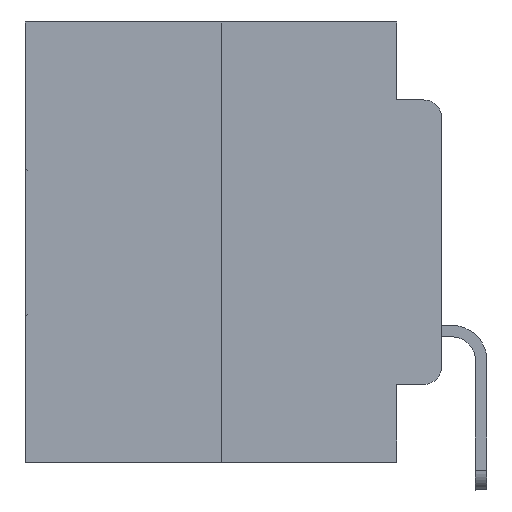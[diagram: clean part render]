
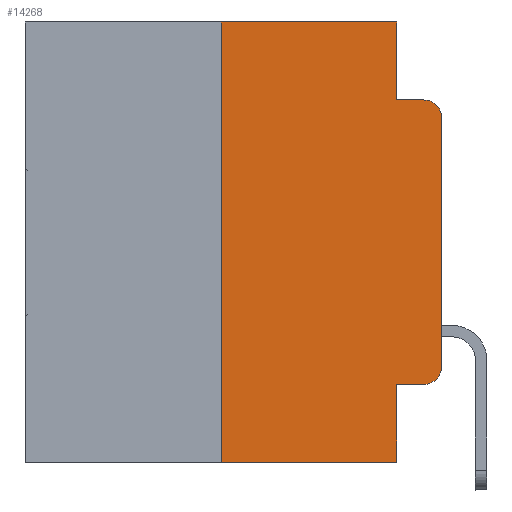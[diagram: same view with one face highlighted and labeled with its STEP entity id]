
A CAD part, left-side view. The second image highlights one B-rep face of the part: STEP entity #14268.
In plain terms, the highlighted planar face has unit normal (-1, 0, 0).
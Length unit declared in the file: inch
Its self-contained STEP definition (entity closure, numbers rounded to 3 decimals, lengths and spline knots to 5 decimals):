
#371 = LINE ( 'NONE', #25552, #9766 ) ;
#422 = CIRCLE ( 'NONE', #6718, 0.02 ) ;
#519 = EDGE_CURVE ( 'NONE', #29199, #28225, #18286, .T. ) ;
#1461 = EDGE_CURVE ( 'NONE', #24950, #4144, #371, .T. ) ;
#1488 = ORIENTED_EDGE ( 'NONE', *, *, #13376, .F. ) ;
#2342 = VECTOR ( 'NONE', #18894, 39.37008 ) ;
#2504 = DIRECTION ( 'NONE',  ( 0., -1., 0. ) ) ;
#2719 = CARTESIAN_POINT ( 'NONE',  ( 0., 0.051, 0. ) ) ;
#3191 = EDGE_CURVE ( 'NONE', #14461, #8366, #22677, .T. ) ;
#3916 = AXIS2_PLACEMENT_3D ( 'NONE', #18688, #4419, #9280 ) ;
#3962 = LINE ( 'NONE', #22178, #16787 ) ;
#4144 = VERTEX_POINT ( 'NONE', #12081 ) ;
#4322 = ORIENTED_EDGE ( 'NONE', *, *, #3191, .F. ) ;
#4419 = DIRECTION ( 'NONE',  ( 1., 0., 0. ) ) ;
#4584 = LINE ( 'NONE', #27183, #28174 ) ;
#5077 = LINE ( 'NONE', #18300, #29204 ) ;
#6096 = DIRECTION ( 'NONE',  ( 0., -1., 0. ) ) ;
#6636 = DIRECTION ( 'NONE',  ( 0., 0., 1. ) ) ;
#6718 = AXIS2_PLACEMENT_3D ( 'NONE', #18452, #28140, #27697 ) ;
#7083 = CARTESIAN_POINT ( 'NONE',  ( 0., 0.051, 0. ) ) ;
#7108 = VERTEX_POINT ( 'NONE', #17450 ) ;
#7921 = ORIENTED_EDGE ( 'NONE', *, *, #13433, .T. ) ;
#8366 = VERTEX_POINT ( 'NONE', #10190 ) ;
#8393 = CARTESIAN_POINT ( 'NONE',  ( 0., 0.02, -0.3915 ) ) ;
#8865 = VECTOR ( 'NONE', #11462, 39.37008 ) ;
#9280 = DIRECTION ( 'NONE',  ( 0., 0., -1. ) ) ;
#9766 = VECTOR ( 'NONE', #6636, 39.37008 ) ;
#9844 = DIRECTION ( 'NONE',  ( 0., 0., -1. ) ) ;
#10190 = CARTESIAN_POINT ( 'NONE',  ( 0., 0.02, -0.0885 ) ) ;
#10726 = EDGE_LOOP ( 'NONE', ( #27563, #7921, #4322, #16764, #29746, #16772, #29697, #1488, #20726, #27313 ) ) ;
#10820 = CARTESIAN_POINT ( 'NONE',  ( 0., 0.051, -0.4115 ) ) ;
#11462 = DIRECTION ( 'NONE',  ( 0., 0., 1. ) ) ;
#12081 = CARTESIAN_POINT ( 'NONE',  ( 0., 0., -0.1085 ) ) ;
#13376 = EDGE_CURVE ( 'NONE', #25265, #7108, #23294, .T. ) ;
#13433 = EDGE_CURVE ( 'NONE', #4144, #8366, #422, .T. ) ;
#14119 = CARTESIAN_POINT ( 'NONE',  ( 0., 0.051, -0.0885 ) ) ;
#14268 = ADVANCED_FACE ( 'NONE', ( #18387 ), #29600, .F. ) ;
#14461 = VERTEX_POINT ( 'NONE', #14119 ) ;
#15403 = VERTEX_POINT ( 'NONE', #29457 ) ;
#15931 = CARTESIAN_POINT ( 'NONE',  ( 0., 0.051, 0. ) ) ;
#15997 = AXIS2_PLACEMENT_3D ( 'NONE', #8393, #26882, #29311 ) ;
#16124 = EDGE_CURVE ( 'NONE', #23951, #14461, #26206, .T. ) ;
#16764 = ORIENTED_EDGE ( 'NONE', *, *, #16124, .F. ) ;
#16772 = ORIENTED_EDGE ( 'NONE', *, *, #519, .F. ) ;
#16787 = VECTOR ( 'NONE', #6096, 39.37008 ) ;
#16794 = EDGE_CURVE ( 'NONE', #15403, #24950, #27704, .T. ) ;
#17091 = VECTOR ( 'NONE', #9844, 39.37008 ) ;
#17124 = EDGE_CURVE ( 'NONE', #28225, #23951, #4584, .T. ) ;
#17450 = CARTESIAN_POINT ( 'NONE',  ( 0., 0.051, -0.5 ) ) ;
#18107 = DIRECTION ( 'NONE',  ( 0., -1., 0. ) ) ;
#18286 = LINE ( 'NONE', #20410, #8865 ) ;
#18300 = CARTESIAN_POINT ( 'NONE',  ( 0., 0.473, -0.5 ) ) ;
#18387 = FACE_OUTER_BOUND ( 'NONE', #10726, .T. ) ;
#18452 = CARTESIAN_POINT ( 'NONE',  ( 0., 0.02, -0.1085 ) ) ;
#18516 = EDGE_CURVE ( 'NONE', #29199, #7108, #5077, .T. ) ;
#18688 = CARTESIAN_POINT ( 'NONE',  ( 0., 0.473, 0. ) ) ;
#18894 = DIRECTION ( 'NONE',  ( 0., 0., -1. ) ) ;
#20409 = DIRECTION ( 'NONE',  ( 0., -1., 0. ) ) ;
#20410 = CARTESIAN_POINT ( 'NONE',  ( 0., 0.25, 0. ) ) ;
#20726 = ORIENTED_EDGE ( 'NONE', *, *, #26731, .T. ) ;
#21582 = CARTESIAN_POINT ( 'NONE',  ( 0., 0., -0.3915 ) ) ;
#22178 = CARTESIAN_POINT ( 'NONE',  ( 0., 0.051, -0.4115 ) ) ;
#22677 = LINE ( 'NONE', #25254, #23213 ) ;
#23213 = VECTOR ( 'NONE', #20409, 39.37008 ) ;
#23294 = LINE ( 'NONE', #7083, #2342 ) ;
#23951 = VERTEX_POINT ( 'NONE', #15931 ) ;
#24516 = CARTESIAN_POINT ( 'NONE',  ( 0., 0.25, -0.5 ) ) ;
#24950 = VERTEX_POINT ( 'NONE', #21582 ) ;
#25254 = CARTESIAN_POINT ( 'NONE',  ( 0., 0.051, -0.0885 ) ) ;
#25265 = VERTEX_POINT ( 'NONE', #10820 ) ;
#25552 = CARTESIAN_POINT ( 'NONE',  ( 0., 0., 0. ) ) ;
#26206 = LINE ( 'NONE', #2719, #17091 ) ;
#26731 = EDGE_CURVE ( 'NONE', #25265, #15403, #3962, .T. ) ;
#26882 = DIRECTION ( 'NONE',  ( -1., 0., 0. ) ) ;
#27183 = CARTESIAN_POINT ( 'NONE',  ( 0., 0.473, 0. ) ) ;
#27313 = ORIENTED_EDGE ( 'NONE', *, *, #16794, .T. ) ;
#27375 = CARTESIAN_POINT ( 'NONE',  ( 0., 0.25, 0. ) ) ;
#27563 = ORIENTED_EDGE ( 'NONE', *, *, #1461, .T. ) ;
#27697 = DIRECTION ( 'NONE',  ( 0., 0., -1. ) ) ;
#27704 = CIRCLE ( 'NONE', #15997, 0.02 ) ;
#28140 = DIRECTION ( 'NONE',  ( -1., 0., 0. ) ) ;
#28174 = VECTOR ( 'NONE', #18107, 39.37008 ) ;
#28225 = VERTEX_POINT ( 'NONE', #27375 ) ;
#29199 = VERTEX_POINT ( 'NONE', #24516 ) ;
#29204 = VECTOR ( 'NONE', #2504, 39.37008 ) ;
#29311 = DIRECTION ( 'NONE',  ( 0., 0., -1. ) ) ;
#29457 = CARTESIAN_POINT ( 'NONE',  ( 0., 0.02, -0.4115 ) ) ;
#29600 = PLANE ( 'NONE',  #3916 ) ;
#29697 = ORIENTED_EDGE ( 'NONE', *, *, #18516, .T. ) ;
#29746 = ORIENTED_EDGE ( 'NONE', *, *, #17124, .F. ) ;
